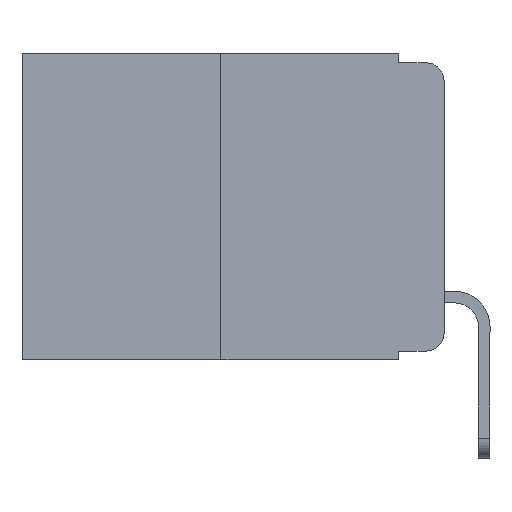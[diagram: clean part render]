
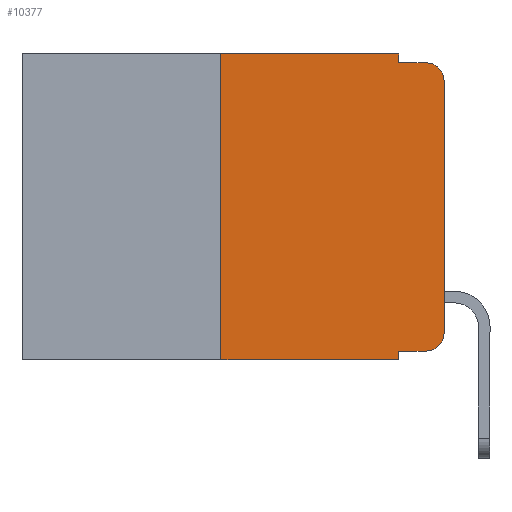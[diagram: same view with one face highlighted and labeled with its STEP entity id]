
A CAD part, left-side view. The second image highlights one B-rep face of the part: STEP entity #10377.
In plain terms, the highlighted planar face has unit normal (-1, 0, 0).
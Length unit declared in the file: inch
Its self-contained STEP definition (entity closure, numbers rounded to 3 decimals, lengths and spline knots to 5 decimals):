
#38 = CARTESIAN_POINT ( 'NONE',  ( 0., 0.051, -0.343 ) ) ;
#299 = CIRCLE ( 'NONE', #9101, 0.02 ) ;
#502 = EDGE_CURVE ( 'NONE', #10356, #988, #4013, .T. ) ;
#574 = EDGE_CURVE ( 'NONE', #988, #2480, #299, .T. ) ;
#599 = EDGE_CURVE ( 'NONE', #10389, #2480, #12150, .T. ) ;
#658 = EDGE_CURVE ( 'NONE', #9791, #10389, #2056, .T. ) ;
#715 = EDGE_LOOP ( 'NONE', ( #5349, #7979, #5685, #5992, #8561, #956, #3680, #8855, #9132, #11705 ) ) ;
#956 = ORIENTED_EDGE ( 'NONE', *, *, #10672, .F. ) ;
#988 = VERTEX_POINT ( 'NONE', #5991 ) ;
#989 = VECTOR ( 'NONE', #4463, 39.37008 ) ;
#1066 = DIRECTION ( 'NONE',  ( 1., 0., 0. ) ) ;
#1159 = CARTESIAN_POINT ( 'NONE',  ( 0., 0.02, -0.01 ) ) ;
#1171 = CARTESIAN_POINT ( 'NONE',  ( 0., 0.02, -0.03 ) ) ;
#1808 = VERTEX_POINT ( 'NONE', #5636 ) ;
#2056 = LINE ( 'NONE', #9313, #11765 ) ;
#2390 = VECTOR ( 'NONE', #2891, 39.37008 ) ;
#2480 = VERTEX_POINT ( 'NONE', #1159 ) ;
#2499 = DIRECTION ( 'NONE',  ( 0., 0., -1. ) ) ;
#2696 = VECTOR ( 'NONE', #11910, 39.37008 ) ;
#2852 = EDGE_CURVE ( 'NONE', #1808, #9791, #10303, .T. ) ;
#2891 = DIRECTION ( 'NONE',  ( 0., -1., 0. ) ) ;
#3118 = CARTESIAN_POINT ( 'NONE',  ( 0., 0.25, -0.343 ) ) ;
#3164 = CARTESIAN_POINT ( 'NONE',  ( 0., 0.051, -0.01 ) ) ;
#3240 = CARTESIAN_POINT ( 'NONE',  ( 0., 0., 0. ) ) ;
#3451 = DIRECTION ( 'NONE',  ( 0., -1., 0. ) ) ;
#3536 = CARTESIAN_POINT ( 'NONE',  ( 0., 0.25, 0. ) ) ;
#3588 = LINE ( 'NONE', #8491, #10567 ) ;
#3680 = ORIENTED_EDGE ( 'NONE', *, *, #9326, .T. ) ;
#4013 = LINE ( 'NONE', #3240, #8616 ) ;
#4057 = CARTESIAN_POINT ( 'NONE',  ( 0., 0.473, 0. ) ) ;
#4189 = CIRCLE ( 'NONE', #11638, 0.02 ) ;
#4463 = DIRECTION ( 'NONE',  ( 0., 0., 1. ) ) ;
#4501 = VERTEX_POINT ( 'NONE', #9767 ) ;
#4760 = VECTOR ( 'NONE', #9270, 39.37008 ) ;
#4952 = LINE ( 'NONE', #8720, #2390 ) ;
#5198 = CARTESIAN_POINT ( 'NONE',  ( 0., 0.02, -0.313 ) ) ;
#5349 = ORIENTED_EDGE ( 'NONE', *, *, #502, .T. ) ;
#5515 = AXIS2_PLACEMENT_3D ( 'NONE', #4057, #1066, #8036 ) ;
#5636 = CARTESIAN_POINT ( 'NONE',  ( 0., 0.25, 0. ) ) ;
#5685 = ORIENTED_EDGE ( 'NONE', *, *, #599, .F. ) ;
#5991 = CARTESIAN_POINT ( 'NONE',  ( 0., 0., -0.03 ) ) ;
#5992 = ORIENTED_EDGE ( 'NONE', *, *, #658, .F. ) ;
#6231 = DIRECTION ( 'NONE',  ( 0., 0., -1. ) ) ;
#6333 = LINE ( 'NONE', #3536, #989 ) ;
#6485 = CARTESIAN_POINT ( 'NONE',  ( 0., 0.473, -0.343 ) ) ;
#7482 = CARTESIAN_POINT ( 'NONE',  ( 0., 0.473, 0. ) ) ;
#7616 = LINE ( 'NONE', #6485, #2696 ) ;
#7656 = VERTEX_POINT ( 'NONE', #38 ) ;
#7660 = EDGE_CURVE ( 'NONE', #10394, #10356, #4189, .T. ) ;
#7868 = DIRECTION ( 'NONE',  ( 0., 0., 1. ) ) ;
#7878 = VECTOR ( 'NONE', #3451, 39.37008 ) ;
#7979 = ORIENTED_EDGE ( 'NONE', *, *, #574, .T. ) ;
#8004 = DIRECTION ( 'NONE',  ( 0., 0., -1. ) ) ;
#8036 = DIRECTION ( 'NONE',  ( 0., 0., -1. ) ) ;
#8491 = CARTESIAN_POINT ( 'NONE',  ( 0., 0.051, 0. ) ) ;
#8561 = ORIENTED_EDGE ( 'NONE', *, *, #2852, .F. ) ;
#8568 = CARTESIAN_POINT ( 'NONE',  ( 0., 0.051, -0.01 ) ) ;
#8616 = VECTOR ( 'NONE', #7868, 39.37008 ) ;
#8720 = CARTESIAN_POINT ( 'NONE',  ( 0., 0.051, -0.333 ) ) ;
#8855 = ORIENTED_EDGE ( 'NONE', *, *, #10100, .F. ) ;
#8892 = EDGE_CURVE ( 'NONE', #4501, #10394, #4952, .T. ) ;
#8929 = PLANE ( 'NONE',  #5515 ) ;
#9101 = AXIS2_PLACEMENT_3D ( 'NONE', #1171, #9116, #8004 ) ;
#9116 = DIRECTION ( 'NONE',  ( -1., 0., 0. ) ) ;
#9132 = ORIENTED_EDGE ( 'NONE', *, *, #8892, .T. ) ;
#9270 = DIRECTION ( 'NONE',  ( 0., -1., 0. ) ) ;
#9313 = CARTESIAN_POINT ( 'NONE',  ( 0., 0.051, 0. ) ) ;
#9326 = EDGE_CURVE ( 'NONE', #10369, #7656, #7616, .T. ) ;
#9767 = CARTESIAN_POINT ( 'NONE',  ( 0., 0.051, -0.333 ) ) ;
#9791 = VERTEX_POINT ( 'NONE', #11033 ) ;
#9870 = CARTESIAN_POINT ( 'NONE',  ( 0., 0.02, -0.333 ) ) ;
#10100 = EDGE_CURVE ( 'NONE', #4501, #7656, #3588, .T. ) ;
#10303 = LINE ( 'NONE', #7482, #7878 ) ;
#10356 = VERTEX_POINT ( 'NONE', #10665 ) ;
#10369 = VERTEX_POINT ( 'NONE', #3118 ) ;
#10377 = ADVANCED_FACE ( 'NONE', ( #11879 ), #8929, .F. ) ;
#10389 = VERTEX_POINT ( 'NONE', #3164 ) ;
#10394 = VERTEX_POINT ( 'NONE', #9870 ) ;
#10567 = VECTOR ( 'NONE', #11974, 39.37008 ) ;
#10665 = CARTESIAN_POINT ( 'NONE',  ( 0., 0., -0.313 ) ) ;
#10672 = EDGE_CURVE ( 'NONE', #10369, #1808, #6333, .T. ) ;
#11033 = CARTESIAN_POINT ( 'NONE',  ( 0., 0.051, 0. ) ) ;
#11638 = AXIS2_PLACEMENT_3D ( 'NONE', #5198, #11678, #6231 ) ;
#11678 = DIRECTION ( 'NONE',  ( -1., 0., 0. ) ) ;
#11705 = ORIENTED_EDGE ( 'NONE', *, *, #7660, .T. ) ;
#11765 = VECTOR ( 'NONE', #2499, 39.37008 ) ;
#11879 = FACE_OUTER_BOUND ( 'NONE', #715, .T. ) ;
#11910 = DIRECTION ( 'NONE',  ( 0., -1., 0. ) ) ;
#11974 = DIRECTION ( 'NONE',  ( 0., 0., -1. ) ) ;
#12150 = LINE ( 'NONE', #8568, #4760 ) ;
